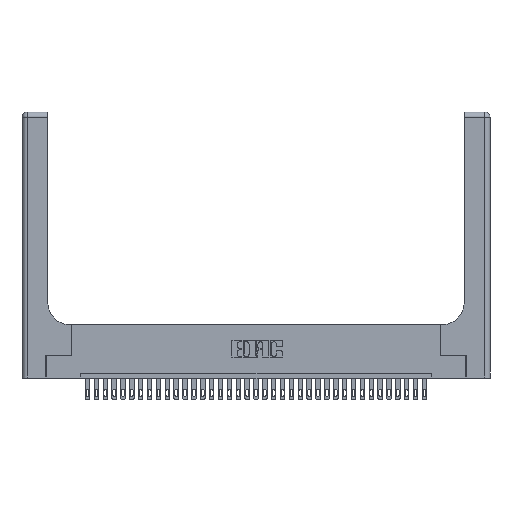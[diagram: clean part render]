
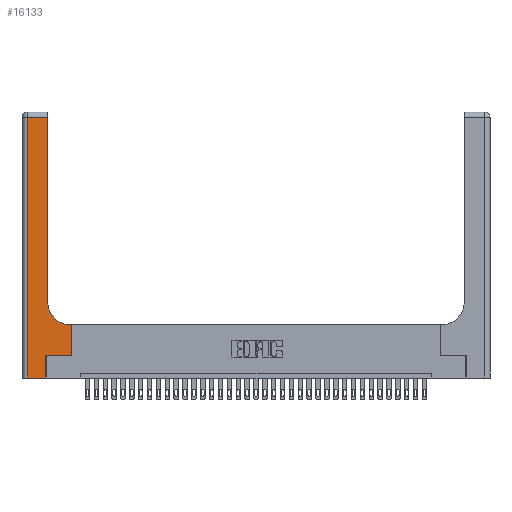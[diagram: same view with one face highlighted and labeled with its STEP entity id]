
A CAD part, top view. The second image highlights one B-rep face of the part: STEP entity #16133.
In plain terms, the highlighted planar face has unit normal (0, 0, 1).
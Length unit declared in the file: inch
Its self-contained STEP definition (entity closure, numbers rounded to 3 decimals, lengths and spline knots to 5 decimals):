
#661 = LINE ( 'NONE', #22731, #17097 ) ;
#665 = VECTOR ( 'NONE', #25022, 39.37008 ) ;
#1043 = DIRECTION ( 'NONE',  ( 0., 1., 0. ) ) ;
#1088 = ORIENTED_EDGE ( 'NONE', *, *, #24154, .T. ) ;
#1089 = DIRECTION ( 'NONE',  ( 0., 0., -1. ) ) ;
#1299 = DIRECTION ( 'NONE',  ( -1., 0., 0. ) ) ;
#1395 = VERTEX_POINT ( 'NONE', #19500 ) ;
#1483 = ORIENTED_EDGE ( 'NONE', *, *, #5510, .T. ) ;
#2115 = CARTESIAN_POINT ( 'NONE',  ( 0., 3., 0.37 ) ) ;
#5510 = EDGE_CURVE ( 'NONE', #33048, #14707, #14524, .T. ) ;
#6144 = LINE ( 'NONE', #13634, #33968 ) ;
#6317 = VERTEX_POINT ( 'NONE', #27856 ) ;
#6469 = EDGE_CURVE ( 'NONE', #31866, #33048, #31685, .T. ) ;
#6681 = CARTESIAN_POINT ( 'NONE',  ( 0.269, 0., 0.37 ) ) ;
#7315 = CARTESIAN_POINT ( 'NONE',  ( 0.2915, 3., 0.37 ) ) ;
#7835 = EDGE_CURVE ( 'NONE', #6317, #23502, #32379, .T. ) ;
#7908 = DIRECTION ( 'NONE',  ( 0., 1., 0. ) ) ;
#8339 = VECTOR ( 'NONE', #7908, 39.37008 ) ;
#8608 = EDGE_CURVE ( 'NONE', #10728, #12563, #14251, .T. ) ;
#8647 = LINE ( 'NONE', #22326, #665 ) ;
#8919 = CARTESIAN_POINT ( 'NONE',  ( 0.269, 0.25, 0.37 ) ) ;
#9428 = DIRECTION ( 'NONE',  ( 1., 0., 0. ) ) ;
#10123 = EDGE_CURVE ( 'NONE', #22998, #1395, #661, .T. ) ;
#10728 = VERTEX_POINT ( 'NONE', #12801 ) ;
#10754 = ORIENTED_EDGE ( 'NONE', *, *, #15532, .T. ) ;
#12210 = ORIENTED_EDGE ( 'NONE', *, *, #8608, .T. ) ;
#12259 = CARTESIAN_POINT ( 'NONE',  ( 0.269, 0., 0.37 ) ) ;
#12563 = VERTEX_POINT ( 'NONE', #25629 ) ;
#12801 = CARTESIAN_POINT ( 'NONE',  ( 0.2915, 0.85, 0.37 ) ) ;
#13030 = CARTESIAN_POINT ( 'NONE',  ( 0.06, 0., 0.37 ) ) ;
#13031 = CIRCLE ( 'NONE', #23556, 0.25 ) ;
#13581 = PLANE ( 'NONE',  #28320 ) ;
#13634 = CARTESIAN_POINT ( 'NONE',  ( 0., 2.94, 0.37 ) ) ;
#13681 = VECTOR ( 'NONE', #9428, 39.37008 ) ;
#13782 = DIRECTION ( 'NONE',  ( 0., 1., 0. ) ) ;
#14251 = LINE ( 'NONE', #7315, #27246 ) ;
#14524 = LINE ( 'NONE', #8919, #13681 ) ;
#14707 = VERTEX_POINT ( 'NONE', #30780 ) ;
#15532 = EDGE_CURVE ( 'NONE', #23502, #31866, #8647, .T. ) ;
#15990 = CARTESIAN_POINT ( 'NONE',  ( 0.5585, 0.6, 0.37 ) ) ;
#16133 = ADVANCED_FACE ( 'NONE', ( #32618 ), #13581, .F. ) ;
#17097 = VECTOR ( 'NONE', #28115, 39.37008 ) ;
#18648 = CARTESIAN_POINT ( 'NONE',  ( 0.5585, 0.25, 0.37 ) ) ;
#18723 = DIRECTION ( 'NONE',  ( 1., 0., 0. ) ) ;
#18979 = EDGE_LOOP ( 'NONE', ( #12210, #32848, #25350, #10754, #32072, #1483, #26280, #27384, #1088 ) ) ;
#19365 = DIRECTION ( 'NONE',  ( 0., -1., 0. ) ) ;
#19500 = CARTESIAN_POINT ( 'NONE',  ( 0.5415, 0.6, 0.37 ) ) ;
#20076 = DIRECTION ( 'NONE',  ( -1., 0., 0. ) ) ;
#20523 = CARTESIAN_POINT ( 'NONE',  ( 0.269, 0.25, 0.37 ) ) ;
#22326 = CARTESIAN_POINT ( 'NONE',  ( 0., 0., 0.37 ) ) ;
#22731 = CARTESIAN_POINT ( 'NONE',  ( 0.2915, 0.6, 0.37 ) ) ;
#22998 = VERTEX_POINT ( 'NONE', #15990 ) ;
#23502 = VERTEX_POINT ( 'NONE', #13030 ) ;
#23556 = AXIS2_PLACEMENT_3D ( 'NONE', #34110, #24004, #18723 ) ;
#24004 = DIRECTION ( 'NONE',  ( 0., 0., -1. ) ) ;
#24154 = EDGE_CURVE ( 'NONE', #1395, #10728, #13031, .T. ) ;
#24482 = VECTOR ( 'NONE', #1043, 39.37008 ) ;
#24904 = CARTESIAN_POINT ( 'NONE',  ( 0.06, 3., 0.37 ) ) ;
#25022 = DIRECTION ( 'NONE',  ( 1., 0., 0. ) ) ;
#25203 = VECTOR ( 'NONE', #19365, 39.37008 ) ;
#25350 = ORIENTED_EDGE ( 'NONE', *, *, #7835, .T. ) ;
#25629 = CARTESIAN_POINT ( 'NONE',  ( 0.2915, 2.94, 0.37 ) ) ;
#26280 = ORIENTED_EDGE ( 'NONE', *, *, #27948, .T. ) ;
#27246 = VECTOR ( 'NONE', #13782, 39.37008 ) ;
#27289 = LINE ( 'NONE', #18648, #8339 ) ;
#27384 = ORIENTED_EDGE ( 'NONE', *, *, #10123, .T. ) ;
#27856 = CARTESIAN_POINT ( 'NONE',  ( 0.06, 2.94, 0.37 ) ) ;
#27948 = EDGE_CURVE ( 'NONE', #14707, #22998, #27289, .T. ) ;
#28115 = DIRECTION ( 'NONE',  ( -1., 0., 0. ) ) ;
#28320 = AXIS2_PLACEMENT_3D ( 'NONE', #2115, #1089, #1299 ) ;
#29941 = EDGE_CURVE ( 'NONE', #12563, #6317, #6144, .T. ) ;
#30780 = CARTESIAN_POINT ( 'NONE',  ( 0.5585, 0.25, 0.37 ) ) ;
#31685 = LINE ( 'NONE', #6681, #24482 ) ;
#31866 = VERTEX_POINT ( 'NONE', #12259 ) ;
#32072 = ORIENTED_EDGE ( 'NONE', *, *, #6469, .T. ) ;
#32379 = LINE ( 'NONE', #24904, #25203 ) ;
#32618 = FACE_OUTER_BOUND ( 'NONE', #18979, .T. ) ;
#32848 = ORIENTED_EDGE ( 'NONE', *, *, #29941, .T. ) ;
#33048 = VERTEX_POINT ( 'NONE', #20523 ) ;
#33968 = VECTOR ( 'NONE', #20076, 39.37008 ) ;
#34110 = CARTESIAN_POINT ( 'NONE',  ( 0.5415, 0.85, 0.37 ) ) ;
